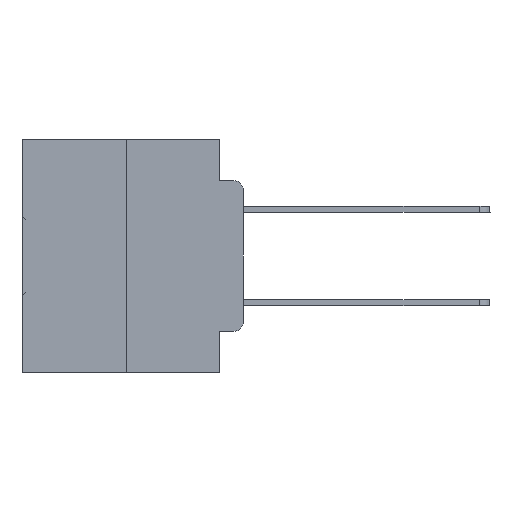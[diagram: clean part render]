
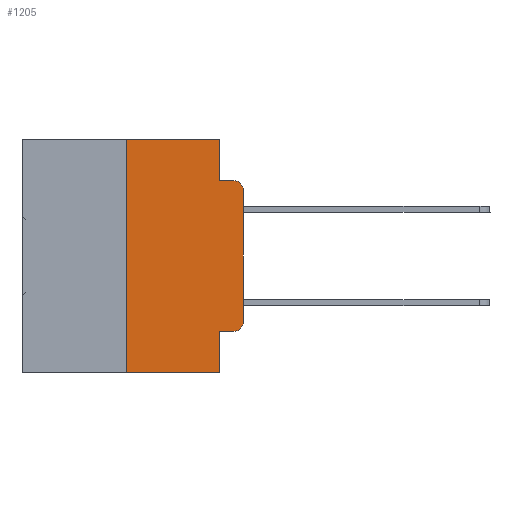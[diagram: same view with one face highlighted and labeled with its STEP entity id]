
A CAD part, left-side view. The second image highlights one B-rep face of the part: STEP entity #1205.
In plain terms, the highlighted planar face has unit normal (-1, 0, 0).
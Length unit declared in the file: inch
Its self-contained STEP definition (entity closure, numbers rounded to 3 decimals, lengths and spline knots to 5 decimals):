
#352 = VERTEX_POINT ( 'NONE', #1380 ) ;
#470 = CARTESIAN_POINT ( 'NONE',  ( 0., 0.051, -0.5 ) ) ;
#625 = CARTESIAN_POINT ( 'NONE',  ( 0., 0.02, -0.3915 ) ) ;
#761 = DIRECTION ( 'NONE',  ( 0., -1., 0. ) ) ;
#1205 = ADVANCED_FACE ( 'NONE', ( #7580 ), #26899, .F. ) ;
#1380 = CARTESIAN_POINT ( 'NONE',  ( 0., 0.051, -0.0885 ) ) ;
#1403 = EDGE_CURVE ( 'NONE', #29198, #352, #29173, .T. ) ;
#1971 = VERTEX_POINT ( 'NONE', #12513 ) ;
#2765 = CARTESIAN_POINT ( 'NONE',  ( 0., 0., -0.3915 ) ) ;
#2902 = ORIENTED_EDGE ( 'NONE', *, *, #19702, .T. ) ;
#2978 = ORIENTED_EDGE ( 'NONE', *, *, #20575, .F. ) ;
#3961 = LINE ( 'NONE', #27225, #22997 ) ;
#4513 = DIRECTION ( 'NONE',  ( 0., 0., -1. ) ) ;
#5816 = VECTOR ( 'NONE', #13359, 39.37008 ) ;
#6005 = EDGE_LOOP ( 'NONE', ( #30142, #20211, #24802, #19516, #26348, #2978, #34945, #27014, #2902, #13071 ) ) ;
#6460 = AXIS2_PLACEMENT_3D ( 'NONE', #625, #25432, #30771 ) ;
#6807 = EDGE_CURVE ( 'NONE', #13352, #7248, #3961, .T. ) ;
#7248 = VERTEX_POINT ( 'NONE', #12014 ) ;
#7261 = EDGE_CURVE ( 'NONE', #26912, #29198, #21720, .T. ) ;
#7395 = CARTESIAN_POINT ( 'NONE',  ( 0., 0.473, 0. ) ) ;
#7521 = DIRECTION ( 'NONE',  ( 0., 0., -1. ) ) ;
#7580 = FACE_OUTER_BOUND ( 'NONE', #6005, .T. ) ;
#7846 = VECTOR ( 'NONE', #30334, 39.37008 ) ;
#8201 = CARTESIAN_POINT ( 'NONE',  ( 0., 0.473, -0.5 ) ) ;
#8490 = AXIS2_PLACEMENT_3D ( 'NONE', #29050, #18190, #4513 ) ;
#9013 = LINE ( 'NONE', #22440, #26796 ) ;
#9271 = VERTEX_POINT ( 'NONE', #16700 ) ;
#9423 = CARTESIAN_POINT ( 'NONE',  ( 0., 0.02, -0.0885 ) ) ;
#9761 = VERTEX_POINT ( 'NONE', #470 ) ;
#10258 = CARTESIAN_POINT ( 'NONE',  ( 0., 0.25, 0. ) ) ;
#10474 = CARTESIAN_POINT ( 'NONE',  ( 0., 0.051, 0. ) ) ;
#12014 = CARTESIAN_POINT ( 'NONE',  ( 0., 0., -0.1085 ) ) ;
#12513 = CARTESIAN_POINT ( 'NONE',  ( 0., 0.02, -0.4115 ) ) ;
#12587 = LINE ( 'NONE', #29930, #31169 ) ;
#13031 = EDGE_CURVE ( 'NONE', #352, #21367, #12587, .T. ) ;
#13071 = ORIENTED_EDGE ( 'NONE', *, *, #35580, .T. ) ;
#13169 = EDGE_CURVE ( 'NONE', #27312, #9761, #32486, .T. ) ;
#13352 = VERTEX_POINT ( 'NONE', #2765 ) ;
#13359 = DIRECTION ( 'NONE',  ( 0., 0., -1. ) ) ;
#13993 = DIRECTION ( 'NONE',  ( 0., 0., -1. ) ) ;
#14567 = CARTESIAN_POINT ( 'NONE',  ( 0., 0.25, -0.5 ) ) ;
#15420 = EDGE_CURVE ( 'NONE', #7248, #21367, #25403, .T. ) ;
#16187 = DIRECTION ( 'NONE',  ( 0., 0., 1. ) ) ;
#16700 = CARTESIAN_POINT ( 'NONE',  ( 0., 0.051, -0.4115 ) ) ;
#17155 = VECTOR ( 'NONE', #761, 39.37008 ) ;
#17290 = CARTESIAN_POINT ( 'NONE',  ( 0., 0.25, 0. ) ) ;
#17927 = DIRECTION ( 'NONE',  ( 0., -1., 0. ) ) ;
#17995 = CIRCLE ( 'NONE', #6460, 0.02 ) ;
#18062 = CARTESIAN_POINT ( 'NONE',  ( 0., 0.473, 0. ) ) ;
#18190 = DIRECTION ( 'NONE',  ( -1., 0., 0. ) ) ;
#19516 = ORIENTED_EDGE ( 'NONE', *, *, #1403, .F. ) ;
#19702 = EDGE_CURVE ( 'NONE', #9271, #1971, #27173, .T. ) ;
#20211 = ORIENTED_EDGE ( 'NONE', *, *, #15420, .T. ) ;
#20575 = EDGE_CURVE ( 'NONE', #27312, #26912, #31371, .T. ) ;
#20842 = VECTOR ( 'NONE', #17927, 39.37008 ) ;
#20940 = DIRECTION ( 'NONE',  ( 1., 0., 0. ) ) ;
#21367 = VERTEX_POINT ( 'NONE', #9423 ) ;
#21720 = LINE ( 'NONE', #18062, #20842 ) ;
#22440 = CARTESIAN_POINT ( 'NONE',  ( 0., 0.051, 0. ) ) ;
#22997 = VECTOR ( 'NONE', #16187, 39.37008 ) ;
#24034 = VECTOR ( 'NONE', #26590, 39.37008 ) ;
#24802 = ORIENTED_EDGE ( 'NONE', *, *, #13031, .F. ) ;
#24942 = AXIS2_PLACEMENT_3D ( 'NONE', #7395, #20940, #7521 ) ;
#25403 = CIRCLE ( 'NONE', #8490, 0.02 ) ;
#25432 = DIRECTION ( 'NONE',  ( -1., 0., 0. ) ) ;
#26348 = ORIENTED_EDGE ( 'NONE', *, *, #7261, .F. ) ;
#26590 = DIRECTION ( 'NONE',  ( 0., 0., 1. ) ) ;
#26796 = VECTOR ( 'NONE', #13993, 39.37008 ) ;
#26899 = PLANE ( 'NONE',  #24942 ) ;
#26912 = VERTEX_POINT ( 'NONE', #17290 ) ;
#27014 = ORIENTED_EDGE ( 'NONE', *, *, #27625, .F. ) ;
#27173 = LINE ( 'NONE', #33892, #17155 ) ;
#27225 = CARTESIAN_POINT ( 'NONE',  ( 0., 0., 0. ) ) ;
#27312 = VERTEX_POINT ( 'NONE', #14567 ) ;
#27625 = EDGE_CURVE ( 'NONE', #9271, #9761, #9013, .T. ) ;
#29050 = CARTESIAN_POINT ( 'NONE',  ( 0., 0.02, -0.1085 ) ) ;
#29173 = LINE ( 'NONE', #10474, #5816 ) ;
#29198 = VERTEX_POINT ( 'NONE', #29894 ) ;
#29894 = CARTESIAN_POINT ( 'NONE',  ( 0., 0.051, 0. ) ) ;
#29930 = CARTESIAN_POINT ( 'NONE',  ( 0., 0.051, -0.0885 ) ) ;
#30142 = ORIENTED_EDGE ( 'NONE', *, *, #6807, .T. ) ;
#30334 = DIRECTION ( 'NONE',  ( 0., -1., 0. ) ) ;
#30771 = DIRECTION ( 'NONE',  ( 0., 0., -1. ) ) ;
#31169 = VECTOR ( 'NONE', #35479, 39.37008 ) ;
#31371 = LINE ( 'NONE', #10258, #24034 ) ;
#32486 = LINE ( 'NONE', #8201, #7846 ) ;
#33892 = CARTESIAN_POINT ( 'NONE',  ( 0., 0.051, -0.4115 ) ) ;
#34945 = ORIENTED_EDGE ( 'NONE', *, *, #13169, .T. ) ;
#35479 = DIRECTION ( 'NONE',  ( 0., -1., 0. ) ) ;
#35580 = EDGE_CURVE ( 'NONE', #1971, #13352, #17995, .T. ) ;
